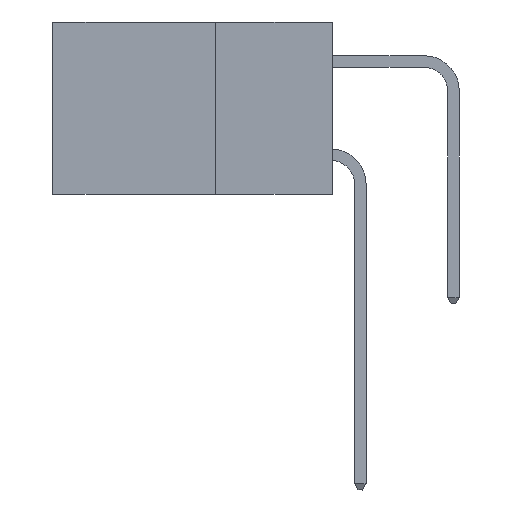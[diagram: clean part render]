
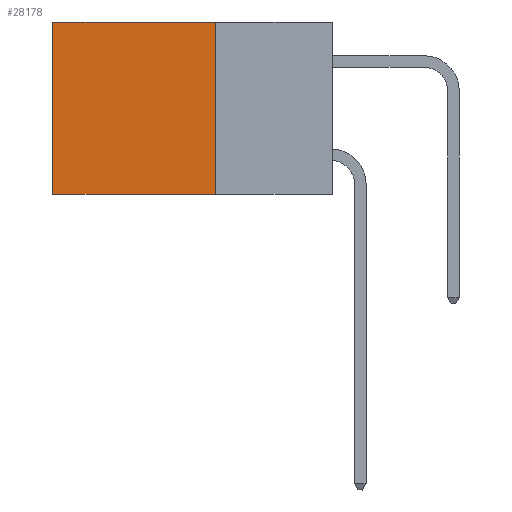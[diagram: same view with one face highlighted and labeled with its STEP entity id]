
A CAD part, left-side view. The second image highlights one B-rep face of the part: STEP entity #28178.
In plain terms, the highlighted planar face has unit normal (-1, 0, 0).
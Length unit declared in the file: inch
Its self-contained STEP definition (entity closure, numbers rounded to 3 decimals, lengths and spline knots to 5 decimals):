
#290 = CARTESIAN_POINT ( 'NONE',  ( 0.298, 0.6, -0.37 ) ) ;
#2220 = DIRECTION ( 'NONE',  ( 0., 0., -1. ) ) ;
#4688 = CARTESIAN_POINT ( 'NONE',  ( 0.298, 0.6, 0. ) ) ;
#6285 = ORIENTED_EDGE ( 'NONE', *, *, #20405, .T. ) ;
#6499 = LINE ( 'NONE', #25148, #15299 ) ;
#6543 = DIRECTION ( 'NONE',  ( 0., 1., 0. ) ) ;
#6971 = PLANE ( 'NONE',  #13145 ) ;
#7356 = FACE_OUTER_BOUND ( 'NONE', #14372, .T. ) ;
#9353 = CARTESIAN_POINT ( 'NONE',  ( 0.298, 0.25, 0. ) ) ;
#9622 = LINE ( 'NONE', #16634, #21855 ) ;
#9660 = VECTOR ( 'NONE', #31269, 39.37008 ) ;
#11185 = VECTOR ( 'NONE', #6543, 39.37008 ) ;
#13145 = AXIS2_PLACEMENT_3D ( 'NONE', #28808, #19273, #24266 ) ;
#13630 = VERTEX_POINT ( 'NONE', #4688 ) ;
#14372 = EDGE_LOOP ( 'NONE', ( #6285, #27812, #23104, #22358 ) ) ;
#14872 = VERTEX_POINT ( 'NONE', #9353 ) ;
#15019 = DIRECTION ( 'NONE',  ( 0., 1., 0. ) ) ;
#15299 = VECTOR ( 'NONE', #15019, 39.37008 ) ;
#15677 = VERTEX_POINT ( 'NONE', #29470 ) ;
#16634 = CARTESIAN_POINT ( 'NONE',  ( 0.298, 0.25, 0. ) ) ;
#19273 = DIRECTION ( 'NONE',  ( 1., 0., 0. ) ) ;
#20405 = EDGE_CURVE ( 'NONE', #13630, #26759, #22641, .T. ) ;
#20497 = EDGE_CURVE ( 'NONE', #14872, #13630, #24555, .T. ) ;
#20595 = EDGE_CURVE ( 'NONE', #14872, #15677, #9622, .T. ) ;
#21770 = EDGE_CURVE ( 'NONE', #15677, #26759, #6499, .T. ) ;
#21855 = VECTOR ( 'NONE', #2220, 39.37008 ) ;
#21929 = CARTESIAN_POINT ( 'NONE',  ( 0.298, 0.25, 0. ) ) ;
#22358 = ORIENTED_EDGE ( 'NONE', *, *, #20497, .T. ) ;
#22641 = LINE ( 'NONE', #26237, #9660 ) ;
#23104 = ORIENTED_EDGE ( 'NONE', *, *, #20595, .F. ) ;
#24266 = DIRECTION ( 'NONE',  ( 0., 0., -1. ) ) ;
#24555 = LINE ( 'NONE', #21929, #11185 ) ;
#25148 = CARTESIAN_POINT ( 'NONE',  ( 0.298, 0.25, -0.37 ) ) ;
#26237 = CARTESIAN_POINT ( 'NONE',  ( 0.298, 0.6, 0. ) ) ;
#26759 = VERTEX_POINT ( 'NONE', #290 ) ;
#27812 = ORIENTED_EDGE ( 'NONE', *, *, #21770, .F. ) ;
#28178 = ADVANCED_FACE ( 'NONE', ( #7356 ), #6971, .F. ) ;
#28808 = CARTESIAN_POINT ( 'NONE',  ( 0.298, 0.25, 0. ) ) ;
#29470 = CARTESIAN_POINT ( 'NONE',  ( 0.298, 0.25, -0.37 ) ) ;
#31269 = DIRECTION ( 'NONE',  ( 0., 0., -1. ) ) ;
